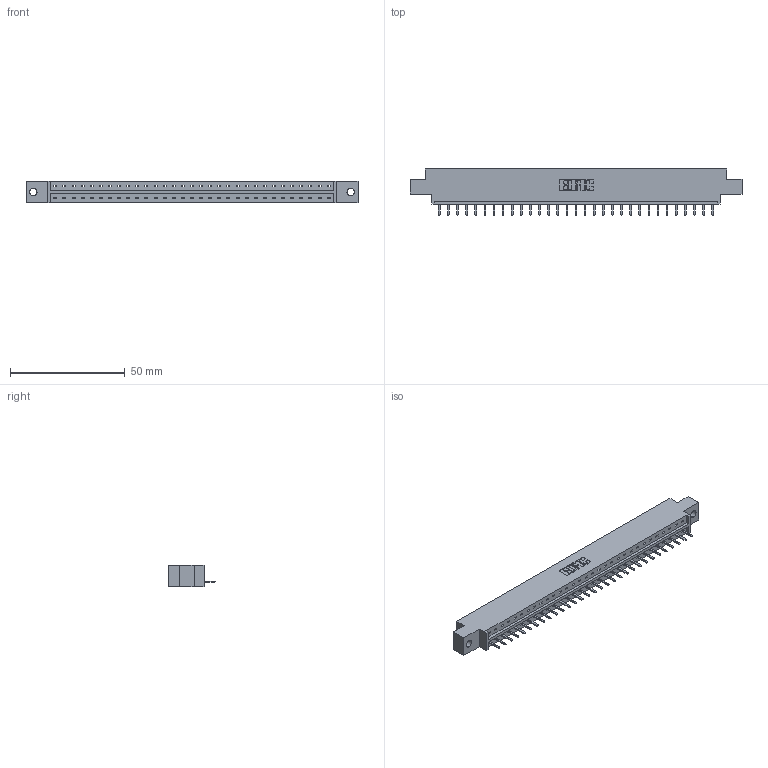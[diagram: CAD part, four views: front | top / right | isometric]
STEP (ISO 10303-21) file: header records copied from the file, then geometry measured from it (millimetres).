
FILE_DESCRIPTION (( 'STEP AP203' ), '1' );
FILE_NAME ('333-031-520-602.STEP', '2018-08-02T19:09:20', ( '' ), ( '' ), 'SwSTEP 2.0', 'SolidWorks 2016', '' );
FILE_SCHEMA (( 'CONFIG_CONTROL_DESIGN' ));
Length unit declared in the file: inch
Products named in the file (3): 333 Part_Offset - .128 Dia; 345-292-001_345-293-120; 333-031-520-602
Assembly tree (32 placements, depth 2):
  333-031-520-602
    333 Part_Offset - .128 Dia
    345-292-001_345-293-120  x31
Bounding box: 144.37 x 20.02 x 9.4 mm (x, y, z)
Volume: 14079.8 mm3; surface area: 14775.1 mm2
Topology: 32 solids, 32 shells, 2040 faces, 6027 edges, 3934 vertices
Faces by surface type: plane 1438, cylinder 602
Entity records: 20623 total; most frequent: CARTESIAN_POINT 3579, ORIENTED_EDGE 3534, DIRECTION 3029, EDGE_CURVE 1767, LINE 1635, VECTOR 1635, VERTEX_POINT 1174, AXIS2_PLACEMENT_3D 697
